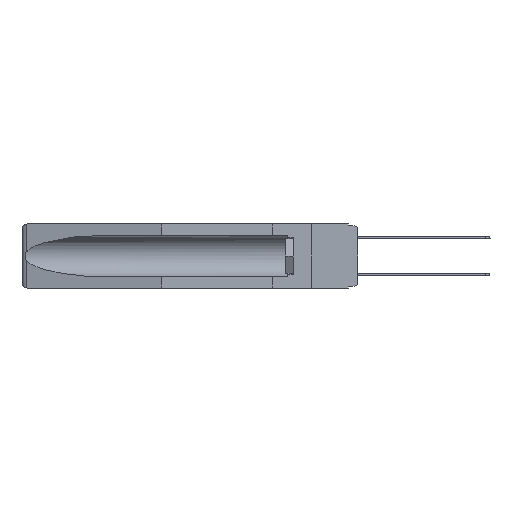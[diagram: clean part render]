
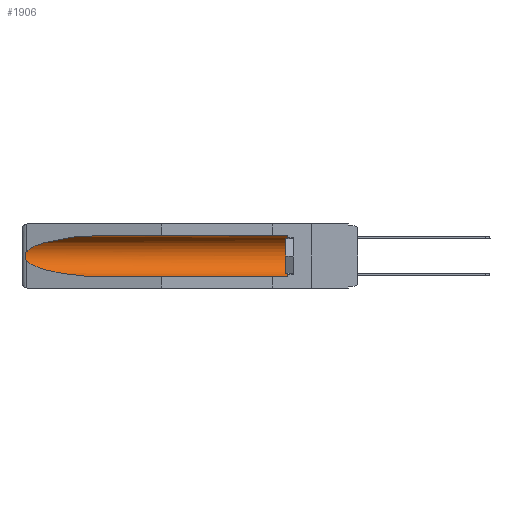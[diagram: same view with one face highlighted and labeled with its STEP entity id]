
A CAD part, left-side view. The second image highlights one B-rep face of the part: STEP entity #1906.
In plain terms, the highlighted cylindrical face has radius 2.857 mm (diameter 5.715 mm), a partial arc.
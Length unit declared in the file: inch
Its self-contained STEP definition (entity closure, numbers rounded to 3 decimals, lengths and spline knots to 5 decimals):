
#756 = CARTESIAN_POINT ( 'NONE',  ( 0.26537, 1.52718, -0.14972 ) ) ;
#1134 = CARTESIAN_POINT ( 'NONE',  ( 0.155, 0.126, -0.1715 ) ) ;
#1767 = VERTEX_POINT ( 'NONE', #12889 ) ;
#1906 = ADVANCED_FACE ( 'NONE', ( #21659 ), #25479, .F. ) ;
#1988 = CARTESIAN_POINT ( 'NONE',  ( 0.21114, 1.30732, -0.284 ) ) ;
#2129 = CARTESIAN_POINT ( 'NONE',  ( 0.155, 1.07973, -0.284 ) ) ;
#2521 = B_SPLINE_CURVE_WITH_KNOTS ( 'NONE', 3,
 ( #14542, #12231, #16290, #24582, #11965, #20357, #12370, #26339, #20638, #18193 ),
 .UNSPECIFIED., .F., .F.,
 ( 4, 2, 2, 2, 4 ),
 ( 0., 0.00029, 0.00058, 0.00087, 0.00117 ),
 .UNSPECIFIED. ) ;
#3043 = EDGE_CURVE ( 'NONE', #1767, #17462, #8583, .T. ) ;
#5625 = CARTESIAN_POINT ( 'NONE',  ( 0.26537, 1.52718, -0.14972 ) ) ;
#7012 = CARTESIAN_POINT ( 'NONE',  ( 0.26537, 1.52718, -0.19328 ) ) ;
#8145 = VERTEX_POINT ( 'NONE', #13640 ) ;
#8260 = CARTESIAN_POINT ( 'NONE',  ( 0.155, 1.07973, -0.284 ) ) ;
#8583 = LINE ( 'NONE', #25487, #24572 ) ;
#9828 = VERTEX_POINT ( 'NONE', #7012 ) ;
#9970 = CARTESIAN_POINT ( 'NONE',  ( 0.25451, 1.48313, -0.24835 ) ) ;
#10368 = VERTEX_POINT ( 'NONE', #5625 ) ;
#10604 = LINE ( 'NONE', #25106, #24952 ) ;
#10955 = AXIS2_PLACEMENT_3D ( 'NONE', #1134, #11957, #20221 ) ;
#10986 = DIRECTION ( 'NONE',  ( 0., 0., 1. ) ) ;
#11248 = ORIENTED_EDGE ( 'NONE', *, *, #25003, .T. ) ;
#11957 = DIRECTION ( 'NONE',  ( 0., -1., 0. ) ) ;
#11965 = CARTESIAN_POINT ( 'NONE',  ( 0.2675, 1.53308, -0.16763 ) ) ;
#12231 = CARTESIAN_POINT ( 'NONE',  ( 0.26597, 1.52961, -0.15275 ) ) ;
#12370 = CARTESIAN_POINT ( 'NONE',  ( 0.2673, 1.53269, -0.17917 ) ) ;
#12378 = AXIS2_PLACEMENT_3D ( 'NONE', #17730, #15554, #10986 ) ;
#12533 = EDGE_CURVE ( 'NONE', #9828, #17462, #17220, .T. ) ;
#12889 = CARTESIAN_POINT ( 'NONE',  ( 0.155, 0.126, -0.284 ) ) ;
#13568 =( BOUNDED_CURVE ( )  B_SPLINE_CURVE ( 3, ( #23905, #25941, #19305, #756 ),
 .UNSPECIFIED., .F., .F. ) 
 B_SPLINE_CURVE_WITH_KNOTS ( ( 4, 4 ),
 ( 4.71239, 6.08839 ),
 .UNSPECIFIED. ) 
 CURVE ( )  GEOMETRIC_REPRESENTATION_ITEM ( )  RATIONAL_B_SPLINE_CURVE ( ( 1., 0.848, 0.848, 1. ) ) 
 REPRESENTATION_ITEM ( '' )  );
#13640 = CARTESIAN_POINT ( 'NONE',  ( 0.155, 1.07973, -0.059 ) ) ;
#14319 = EDGE_CURVE ( 'NONE', #10368, #9828, #2521, .T. ) ;
#14422 = CIRCLE ( 'NONE', #10955, 0.1125 ) ;
#14423 = EDGE_CURVE ( 'NONE', #18995, #8145, #10604, .T. ) ;
#14542 = CARTESIAN_POINT ( 'NONE',  ( 0.26537, 1.52718, -0.14972 ) ) ;
#15120 = CARTESIAN_POINT ( 'NONE',  ( 0.155, 0.126, -0.059 ) ) ;
#15554 = DIRECTION ( 'NONE',  ( 0., 1., 0. ) ) ;
#16290 = CARTESIAN_POINT ( 'NONE',  ( 0.26654, 1.53092, -0.15636 ) ) ;
#16813 = DIRECTION ( 'NONE',  ( 0., 1., 0. ) ) ;
#17220 =( BOUNDED_CURVE ( )  B_SPLINE_CURVE ( 3, ( #26494, #9970, #1988, #2129 ),
 .UNSPECIFIED., .F., .F. ) 
 B_SPLINE_CURVE_WITH_KNOTS ( ( 4, 4 ),
 ( 0.1948, 1.5708 ),
 .UNSPECIFIED. ) 
 CURVE ( )  GEOMETRIC_REPRESENTATION_ITEM ( )  RATIONAL_B_SPLINE_CURVE ( ( 1., 0.848, 0.848, 1. ) ) 
 REPRESENTATION_ITEM ( '' )  );
#17462 = VERTEX_POINT ( 'NONE', #8260 ) ;
#17730 = CARTESIAN_POINT ( 'NONE',  ( 0.155, -0.30754, -0.1715 ) ) ;
#18193 = CARTESIAN_POINT ( 'NONE',  ( 0.26537, 1.52718, -0.19328 ) ) ;
#18807 = ORIENTED_EDGE ( 'NONE', *, *, #14423, .T. ) ;
#18862 = DIRECTION ( 'NONE',  ( 0., 1., 0. ) ) ;
#18995 = VERTEX_POINT ( 'NONE', #15120 ) ;
#19269 = EDGE_LOOP ( 'NONE', ( #22958, #25324, #20881, #19888, #11248, #18807 ) ) ;
#19305 = CARTESIAN_POINT ( 'NONE',  ( 0.25451, 1.48313, -0.09465 ) ) ;
#19888 = ORIENTED_EDGE ( 'NONE', *, *, #3043, .F. ) ;
#20221 = DIRECTION ( 'NONE',  ( 0., 0., 1. ) ) ;
#20357 = CARTESIAN_POINT ( 'NONE',  ( 0.2675, 1.53308, -0.17534 ) ) ;
#20638 = CARTESIAN_POINT ( 'NONE',  ( 0.26597, 1.5296, -0.19026 ) ) ;
#20816 = EDGE_CURVE ( 'NONE', #8145, #10368, #13568, .T. ) ;
#20881 = ORIENTED_EDGE ( 'NONE', *, *, #12533, .T. ) ;
#21659 = FACE_OUTER_BOUND ( 'NONE', #19269, .T. ) ;
#22958 = ORIENTED_EDGE ( 'NONE', *, *, #20816, .T. ) ;
#23905 = CARTESIAN_POINT ( 'NONE',  ( 0.155, 1.07973, -0.059 ) ) ;
#24572 = VECTOR ( 'NONE', #16813, 39.37008 ) ;
#24582 = CARTESIAN_POINT ( 'NONE',  ( 0.2673, 1.5327, -0.16383 ) ) ;
#24952 = VECTOR ( 'NONE', #18862, 39.37008 ) ;
#25003 = EDGE_CURVE ( 'NONE', #1767, #18995, #14422, .T. ) ;
#25106 = CARTESIAN_POINT ( 'NONE',  ( 0.155, -0.30754, -0.059 ) ) ;
#25324 = ORIENTED_EDGE ( 'NONE', *, *, #14319, .T. ) ;
#25479 = CYLINDRICAL_SURFACE ( 'NONE', #12378, 0.1125 ) ;
#25487 = CARTESIAN_POINT ( 'NONE',  ( 0.155, -0.30754, -0.284 ) ) ;
#25941 = CARTESIAN_POINT ( 'NONE',  ( 0.21114, 1.30732, -0.059 ) ) ;
#26339 = CARTESIAN_POINT ( 'NONE',  ( 0.26655, 1.53094, -0.18657 ) ) ;
#26494 = CARTESIAN_POINT ( 'NONE',  ( 0.26537, 1.52718, -0.19328 ) ) ;
